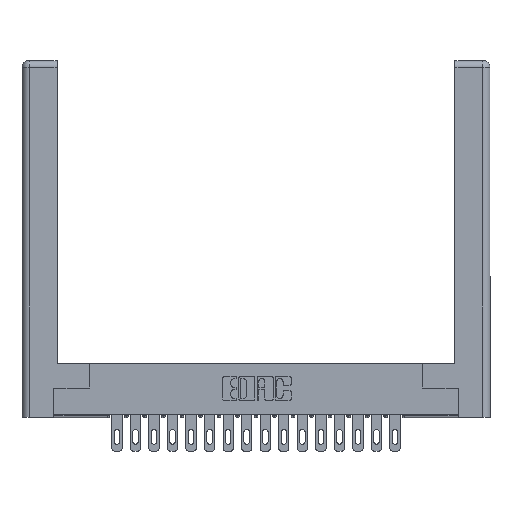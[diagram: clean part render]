
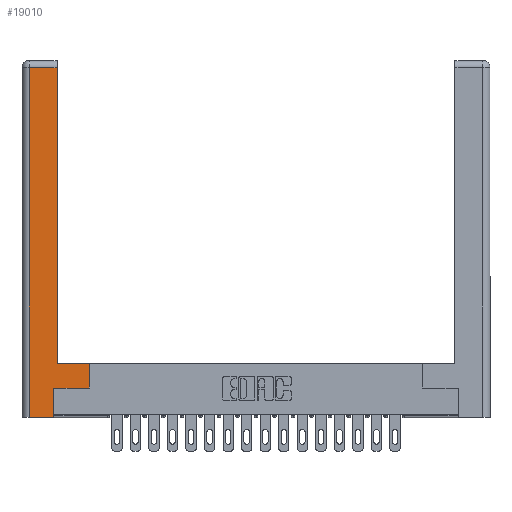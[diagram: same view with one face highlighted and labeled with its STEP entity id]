
A CAD part, top view. The second image highlights one B-rep face of the part: STEP entity #19010.
In plain terms, the highlighted planar face has unit normal (0, 0, 1).
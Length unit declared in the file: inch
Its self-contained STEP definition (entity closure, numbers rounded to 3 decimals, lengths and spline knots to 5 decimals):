
#675 = CARTESIAN_POINT ( 'NONE',  ( 0.295, 0.45, 0. ) ) ;
#826 = CARTESIAN_POINT ( 'NONE',  ( 0.0615, 0., 0. ) ) ;
#1197 = EDGE_CURVE ( 'NONE', #9194, #21083, #7909, .T. ) ;
#1566 = VECTOR ( 'NONE', #8532, 39.37008 ) ;
#1631 = CARTESIAN_POINT ( 'NONE',  ( 0.295, 3., 0. ) ) ;
#1776 = EDGE_CURVE ( 'NONE', #19272, #5865, #10573, .T. ) ;
#2154 = ORIENTED_EDGE ( 'NONE', *, *, #1197, .T. ) ;
#2680 = EDGE_CURVE ( 'NONE', #17054, #16930, #13668, .T. ) ;
#3282 = LINE ( 'NONE', #1631, #19924 ) ;
#3379 = VECTOR ( 'NONE', #17417, 39.37008 ) ;
#3536 = ORIENTED_EDGE ( 'NONE', *, *, #17495, .T. ) ;
#4278 = CARTESIAN_POINT ( 'NONE',  ( 0.265, 0., 0. ) ) ;
#4955 = EDGE_CURVE ( 'NONE', #10443, #19272, #10422, .T. ) ;
#5395 = ORIENTED_EDGE ( 'NONE', *, *, #18765, .T. ) ;
#5865 = VERTEX_POINT ( 'NONE', #675 ) ;
#5935 = ORIENTED_EDGE ( 'NONE', *, *, #8469, .T. ) ;
#6428 = EDGE_LOOP ( 'NONE', ( #15206, #5935, #11481, #5395, #2154, #3536, #16465, #10512 ) ) ;
#7167 = LINE ( 'NONE', #17118, #10891 ) ;
#7235 = CARTESIAN_POINT ( 'NONE',  ( 0.265, 0.245, 0. ) ) ;
#7644 = DIRECTION ( 'NONE',  ( 0., -1., 0. ) ) ;
#7909 = LINE ( 'NONE', #7235, #3379 ) ;
#7922 = VECTOR ( 'NONE', #20374, 39.37008 ) ;
#8254 = CARTESIAN_POINT ( 'NONE',  ( 0., 0., 0. ) ) ;
#8338 = LINE ( 'NONE', #14810, #16259 ) ;
#8469 = EDGE_CURVE ( 'NONE', #15150, #17054, #8338, .T. ) ;
#8532 = DIRECTION ( 'NONE',  ( 0., 1., 0. ) ) ;
#8569 = CARTESIAN_POINT ( 'NONE',  ( 0.265, 0.245, 0. ) ) ;
#8880 = LINE ( 'NONE', #4278, #7922 ) ;
#9018 = CARTESIAN_POINT ( 'NONE',  ( 0.0615, 0., 0. ) ) ;
#9194 = VERTEX_POINT ( 'NONE', #19804 ) ;
#9665 = EDGE_CURVE ( 'NONE', #5865, #15150, #3282, .T. ) ;
#9853 = DIRECTION ( 'NONE',  ( -1., 0., 0. ) ) ;
#10422 = LINE ( 'NONE', #14775, #1566 ) ;
#10443 = VERTEX_POINT ( 'NONE', #13521 ) ;
#10512 = ORIENTED_EDGE ( 'NONE', *, *, #1776, .T. ) ;
#10573 = LINE ( 'NONE', #13524, #18524 ) ;
#10891 = VECTOR ( 'NONE', #17041, 39.37008 ) ;
#11481 = ORIENTED_EDGE ( 'NONE', *, *, #2680, .T. ) ;
#13425 = CARTESIAN_POINT ( 'NONE',  ( 0.565, 0.45, 0. ) ) ;
#13521 = CARTESIAN_POINT ( 'NONE',  ( 0.565, 0.245, 0. ) ) ;
#13524 = CARTESIAN_POINT ( 'NONE',  ( 0.295, 0.45, 0. ) ) ;
#13660 = DIRECTION ( 'NONE',  ( -1., 0., 0. ) ) ;
#13668 = LINE ( 'NONE', #826, #17490 ) ;
#14072 = CARTESIAN_POINT ( 'NONE',  ( 0.0615, 2.94, 0. ) ) ;
#14517 = FACE_OUTER_BOUND ( 'NONE', #6428, .T. ) ;
#14775 = CARTESIAN_POINT ( 'NONE',  ( 0.565, 0.45, 0. ) ) ;
#14810 = CARTESIAN_POINT ( 'NONE',  ( 0.0615, 2.94, 0. ) ) ;
#15150 = VERTEX_POINT ( 'NONE', #15161 ) ;
#15161 = CARTESIAN_POINT ( 'NONE',  ( 0.295, 2.94, 0. ) ) ;
#15206 = ORIENTED_EDGE ( 'NONE', *, *, #9665, .T. ) ;
#16137 = PLANE ( 'NONE',  #17355 ) ;
#16259 = VECTOR ( 'NONE', #16457, 39.37008 ) ;
#16336 = DIRECTION ( 'NONE',  ( 0., 1., 0. ) ) ;
#16457 = DIRECTION ( 'NONE',  ( -1., 0., 0. ) ) ;
#16465 = ORIENTED_EDGE ( 'NONE', *, *, #4955, .T. ) ;
#16930 = VERTEX_POINT ( 'NONE', #9018 ) ;
#17041 = DIRECTION ( 'NONE',  ( 1., 0., 0. ) ) ;
#17054 = VERTEX_POINT ( 'NONE', #14072 ) ;
#17118 = CARTESIAN_POINT ( 'NONE',  ( 0.565, 0.245, 0. ) ) ;
#17355 = AXIS2_PLACEMENT_3D ( 'NONE', #8254, #19316, #9853 ) ;
#17417 = DIRECTION ( 'NONE',  ( 0., 1., 0. ) ) ;
#17490 = VECTOR ( 'NONE', #7644, 39.37008 ) ;
#17495 = EDGE_CURVE ( 'NONE', #21083, #10443, #7167, .T. ) ;
#18524 = VECTOR ( 'NONE', #13660, 39.37008 ) ;
#18765 = EDGE_CURVE ( 'NONE', #16930, #9194, #8880, .T. ) ;
#19010 = ADVANCED_FACE ( 'NONE', ( #14517 ), #16137, .F. ) ;
#19272 = VERTEX_POINT ( 'NONE', #13425 ) ;
#19316 = DIRECTION ( 'NONE',  ( 0., 0., -1. ) ) ;
#19804 = CARTESIAN_POINT ( 'NONE',  ( 0.265, 0., 0. ) ) ;
#19924 = VECTOR ( 'NONE', #16336, 39.37008 ) ;
#20374 = DIRECTION ( 'NONE',  ( 1., 0., 0. ) ) ;
#21083 = VERTEX_POINT ( 'NONE', #8569 ) ;
